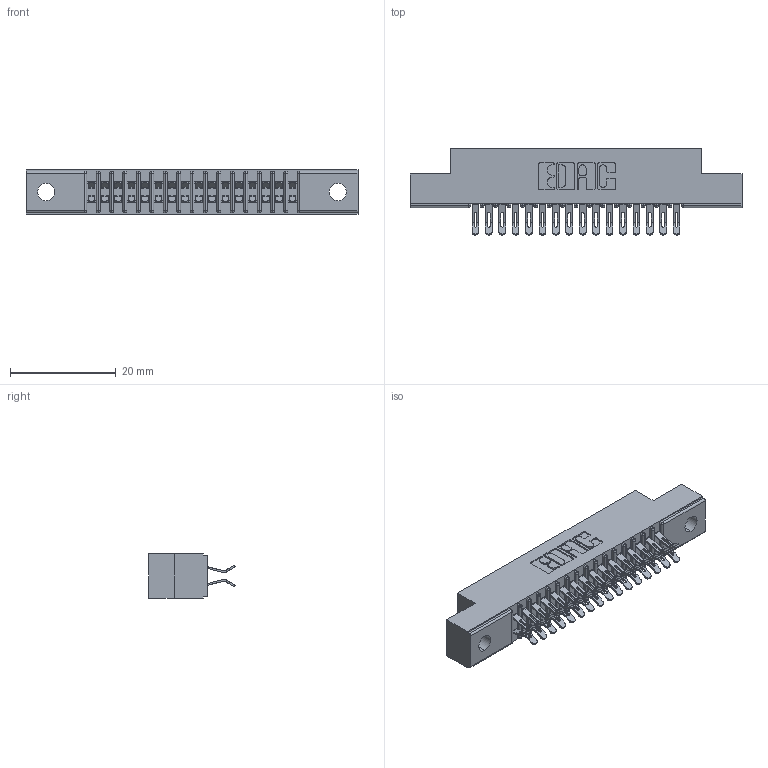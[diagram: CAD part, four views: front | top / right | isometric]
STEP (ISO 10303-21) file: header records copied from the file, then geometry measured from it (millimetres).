
FILE_DESCRIPTION (( 'STEP AP203' ), '1' );
FILE_NAME ('391-032-555-202.STEP', '2018-08-08T22:17:29', ( '' ), ( '' ), 'SwSTEP 2.0', 'SolidWorks 2016', '' );
FILE_SCHEMA (( 'CONFIG_CONTROL_DESIGN' ));
Length unit declared in the file: inch
Products named in the file (3): 341 Part_.128 (3.25) Dia Mounting Holes; 341-292-001_341-292-155; 391-032-555-202
Assembly tree (33 placements, depth 2):
  391-032-555-202
    341 Part_.128 (3.25) Dia Mounting Holes
    341-292-001_341-292-155  x32
Bounding box: 62.87 x 16.31 x 8.38 mm (x, y, z)
Volume: 3595.9 mm3; surface area: 7130.1 mm2
Topology: 33 solids, 33 shells, 2612 faces, 7788 edges, 5070 vertices
Faces by surface type: plane 1412, cylinder 1136, sphere 34, torus 30
Entity records: 23299 total; most frequent: CARTESIAN_POINT 3890, ORIENTED_EDGE 3852, DIRECTION 3784, EDGE_CURVE 1926, LINE 1512, VECTOR 1512, VERTEX_POINT 1226, AXIS2_PLACEMENT_3D 1136
